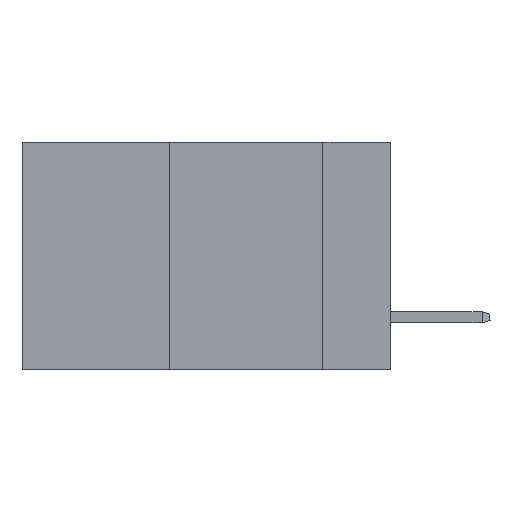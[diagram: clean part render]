
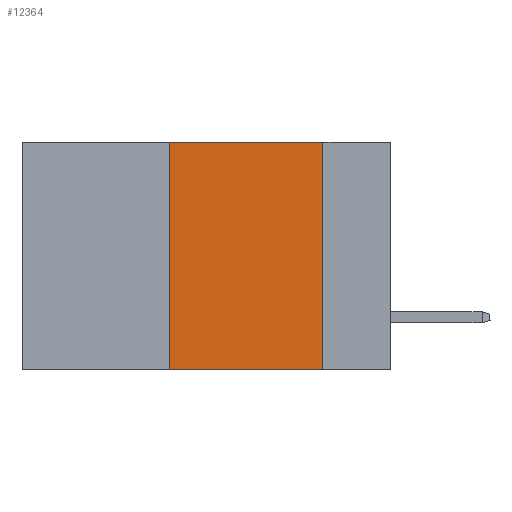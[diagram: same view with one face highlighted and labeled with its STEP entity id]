
A CAD part, left-side view. The second image highlights one B-rep face of the part: STEP entity #12364.
In plain terms, the highlighted planar face has unit normal (-1, 0, 0).
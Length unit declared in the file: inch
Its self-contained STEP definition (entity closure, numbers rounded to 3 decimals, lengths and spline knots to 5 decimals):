
#161 = CARTESIAN_POINT ( 'NONE',  ( 0., 0.11, 0. ) ) ;
#556 = VERTEX_POINT ( 'NONE', #21454 ) ;
#930 = EDGE_CURVE ( 'NONE', #556, #16173, #5915, .T. ) ;
#1531 = VERTEX_POINT ( 'NONE', #21056 ) ;
#1859 = DIRECTION ( 'NONE',  ( 0., 0., -1. ) ) ;
#2778 = AXIS2_PLACEMENT_3D ( 'NONE', #8815, #14009, #20702 ) ;
#3527 = CARTESIAN_POINT ( 'NONE',  ( 0., 0.6, 0. ) ) ;
#3539 = CARTESIAN_POINT ( 'NONE',  ( 0., 0.36, -0.37 ) ) ;
#3546 = EDGE_CURVE ( 'NONE', #14914, #1531, #12932, .T. ) ;
#3715 = VECTOR ( 'NONE', #1859, 39.37008 ) ;
#5915 = LINE ( 'NONE', #3527, #12505 ) ;
#5951 = FACE_OUTER_BOUND ( 'NONE', #13108, .T. ) ;
#8417 = DIRECTION ( 'NONE',  ( 0., -1., 0. ) ) ;
#8739 = PLANE ( 'NONE',  #2778 ) ;
#8815 = CARTESIAN_POINT ( 'NONE',  ( 0., 0.6, 0. ) ) ;
#9201 = DIRECTION ( 'NONE',  ( 0., -1., 0. ) ) ;
#9218 = CARTESIAN_POINT ( 'NONE',  ( 0., 0.36, 0. ) ) ;
#9699 = ORIENTED_EDGE ( 'NONE', *, *, #930, .F. ) ;
#9788 = LINE ( 'NONE', #161, #3715 ) ;
#12364 = ADVANCED_FACE ( 'NONE', ( #5951 ), #8739, .F. ) ;
#12505 = VECTOR ( 'NONE', #8417, 39.37008 ) ;
#12932 = LINE ( 'NONE', #21038, #20368 ) ;
#13108 = EDGE_LOOP ( 'NONE', ( #17111, #9699, #13533, #20960 ) ) ;
#13466 = EDGE_CURVE ( 'NONE', #14914, #556, #21278, .T. ) ;
#13533 = ORIENTED_EDGE ( 'NONE', *, *, #13466, .F. ) ;
#14009 = DIRECTION ( 'NONE',  ( 1., 0., 0. ) ) ;
#14914 = VERTEX_POINT ( 'NONE', #3539 ) ;
#15074 = EDGE_CURVE ( 'NONE', #16173, #1531, #9788, .T. ) ;
#16173 = VERTEX_POINT ( 'NONE', #21658 ) ;
#17111 = ORIENTED_EDGE ( 'NONE', *, *, #15074, .F. ) ;
#17340 = DIRECTION ( 'NONE',  ( 0., 0., 1. ) ) ;
#20368 = VECTOR ( 'NONE', #9201, 39.37008 ) ;
#20702 = DIRECTION ( 'NONE',  ( 0., 0., -1. ) ) ;
#20960 = ORIENTED_EDGE ( 'NONE', *, *, #3546, .T. ) ;
#21038 = CARTESIAN_POINT ( 'NONE',  ( 0., 0.6, -0.37 ) ) ;
#21056 = CARTESIAN_POINT ( 'NONE',  ( 0., 0.11, -0.37 ) ) ;
#21278 = LINE ( 'NONE', #9218, #21817 ) ;
#21454 = CARTESIAN_POINT ( 'NONE',  ( 0., 0.36, 0. ) ) ;
#21658 = CARTESIAN_POINT ( 'NONE',  ( 0., 0.11, 0. ) ) ;
#21817 = VECTOR ( 'NONE', #17340, 39.37008 ) ;
